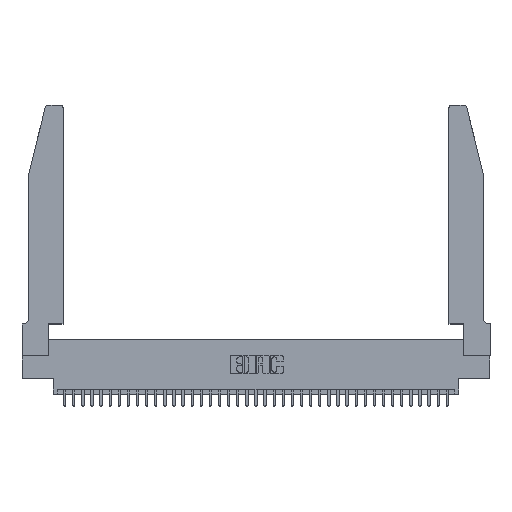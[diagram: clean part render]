
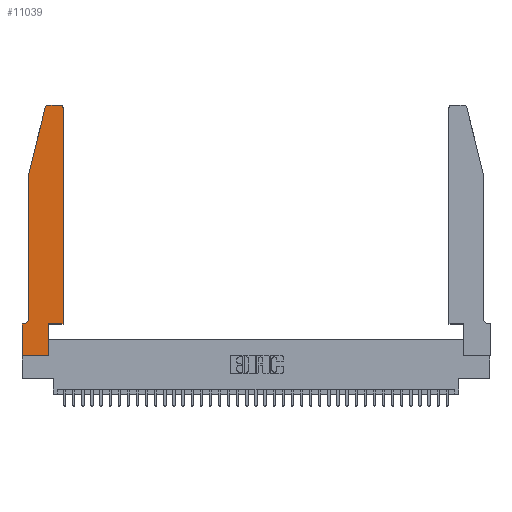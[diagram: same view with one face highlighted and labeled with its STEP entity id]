
A CAD part, top view. The second image highlights one B-rep face of the part: STEP entity #11039.
In plain terms, the highlighted planar face has unit normal (0, 0, 1).
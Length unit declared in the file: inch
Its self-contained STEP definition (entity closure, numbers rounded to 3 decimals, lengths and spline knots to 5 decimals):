
#48 = ORIENTED_EDGE ( 'NONE', *, *, #18609, .T. ) ;
#367 = ORIENTED_EDGE ( 'NONE', *, *, #29349, .T. ) ;
#1250 = CARTESIAN_POINT ( 'NONE',  ( 0.0755, 0.42, 0.37 ) ) ;
#1314 = VECTOR ( 'NONE', #4894, 39.37008 ) ;
#1820 = DIRECTION ( 'NONE',  ( -1., 0., 0. ) ) ;
#1969 = VERTEX_POINT ( 'NONE', #32398 ) ;
#2096 = LINE ( 'NONE', #29753, #17162 ) ;
#2302 = AXIS2_PLACEMENT_3D ( 'NONE', #9084, #29878, #12123 ) ;
#3725 = LINE ( 'NONE', #3844, #17818 ) ;
#3844 = CARTESIAN_POINT ( 'NONE',  ( 0., 0., 0.37 ) ) ;
#4588 = VECTOR ( 'NONE', #27755, 39.37008 ) ;
#4894 = DIRECTION ( 'NONE',  ( 0., 1., 0. ) ) ;
#4988 = VERTEX_POINT ( 'NONE', #13784 ) ;
#5032 = VERTEX_POINT ( 'NONE', #22776 ) ;
#5571 = CARTESIAN_POINT ( 'NONE',  ( 0.0755, 2., 0.37 ) ) ;
#5693 = CARTESIAN_POINT ( 'NONE',  ( 0., 0.35, 0.37 ) ) ;
#6256 = CARTESIAN_POINT ( 'NONE',  ( 0.4205, 2.72, 0.37 ) ) ;
#6925 = CARTESIAN_POINT ( 'NONE',  ( 0., 0., 0.37 ) ) ;
#7470 = EDGE_CURVE ( 'NONE', #35418, #28809, #28387, .T. ) ;
#8355 = ORIENTED_EDGE ( 'NONE', *, *, #7470, .T. ) ;
#8602 = LINE ( 'NONE', #31963, #14700 ) ;
#8677 = VECTOR ( 'NONE', #22527, 39.37008 ) ;
#8718 = DIRECTION ( 'NONE',  ( 0., 0., 1. ) ) ;
#9068 = AXIS2_PLACEMENT_3D ( 'NONE', #28570, #10781, #31528 ) ;
#9084 = CARTESIAN_POINT ( 'NONE',  ( 0.0055, 0.42, 0.37 ) ) ;
#9276 = DIRECTION ( 'NONE',  ( 1., 0., 0. ) ) ;
#9412 = CIRCLE ( 'NONE', #9068, 0.03 ) ;
#9448 = VERTEX_POINT ( 'NONE', #37239 ) ;
#10198 = EDGE_CURVE ( 'NONE', #10254, #31013, #8602, .T. ) ;
#10254 = VERTEX_POINT ( 'NONE', #5571 ) ;
#10673 = EDGE_CURVE ( 'NONE', #4988, #35418, #16707, .T. ) ;
#10781 = DIRECTION ( 'NONE',  ( 0., 0., 1. ) ) ;
#10873 = EDGE_CURVE ( 'NONE', #1969, #31015, #2096, .T. ) ;
#11039 = ADVANCED_FACE ( 'NONE', ( #13440 ), #23602, .T. ) ;
#11080 = CARTESIAN_POINT ( 'NONE',  ( 0.0755, 0.35, 0.37 ) ) ;
#12123 = DIRECTION ( 'NONE',  ( -1., 0., 0. ) ) ;
#13274 = CARTESIAN_POINT ( 'NONE',  ( 0.4505, 0.35, 0.37 ) ) ;
#13440 = FACE_OUTER_BOUND ( 'NONE', #13988, .T. ) ;
#13545 = CARTESIAN_POINT ( 'NONE',  ( 0.2605, 2.75, 0.37 ) ) ;
#13784 = CARTESIAN_POINT ( 'NONE',  ( 0.0055, 0.35, 0.37 ) ) ;
#13850 = CARTESIAN_POINT ( 'NONE',  ( 0.0755, 2., 0.37 ) ) ;
#13942 = ORIENTED_EDGE ( 'NONE', *, *, #18592, .T. ) ;
#13988 = EDGE_LOOP ( 'NONE', ( #367, #29294, #13942, #35464, #27269, #30937, #8355, #35736, #48, #34178, #27281, #27553 ) ) ;
#14250 = DIRECTION ( 'NONE',  ( 0., -1., 0. ) ) ;
#14700 = VECTOR ( 'NONE', #14250, 39.37008 ) ;
#14840 = EDGE_CURVE ( 'NONE', #9448, #34314, #9412, .T. ) ;
#16391 = LINE ( 'NONE', #28755, #1314 ) ;
#16707 = LINE ( 'NONE', #11080, #31525 ) ;
#16716 = EDGE_CURVE ( 'NONE', #31015, #5032, #37943, .T. ) ;
#17093 = EDGE_CURVE ( 'NONE', #31013, #4988, #34979, .T. ) ;
#17162 = VECTOR ( 'NONE', #32703, 39.37008 ) ;
#17196 = CARTESIAN_POINT ( 'NONE',  ( 0., 0., 0.37 ) ) ;
#17292 = CARTESIAN_POINT ( 'NONE',  ( 0.4505, 0.35, 0.37 ) ) ;
#17818 = VECTOR ( 'NONE', #24779, 39.37008 ) ;
#18349 = EDGE_CURVE ( 'NONE', #28809, #25086, #3725, .T. ) ;
#18592 = EDGE_CURVE ( 'NONE', #34314, #10254, #33052, .T. ) ;
#18609 = EDGE_CURVE ( 'NONE', #25086, #1969, #16391, .T. ) ;
#22527 = DIRECTION ( 'NONE',  ( -1., 0., 0. ) ) ;
#22776 = CARTESIAN_POINT ( 'NONE',  ( 0.4505, 2.72, 0.37 ) ) ;
#23157 = EDGE_CURVE ( 'NONE', #5032, #29342, #26316, .T. ) ;
#23602 = PLANE ( 'NONE',  #35067 ) ;
#24428 = CARTESIAN_POINT ( 'NONE',  ( 0.2865, 0., 0.37 ) ) ;
#24779 = DIRECTION ( 'NONE',  ( 1., 0., 0. ) ) ;
#25086 = VERTEX_POINT ( 'NONE', #24428 ) ;
#25229 = VECTOR ( 'NONE', #28625, 39.37008 ) ;
#26316 = CIRCLE ( 'NONE', #34104, 0.03 ) ;
#27121 = DIRECTION ( 'NONE',  ( 0., 0., 1. ) ) ;
#27269 = ORIENTED_EDGE ( 'NONE', *, *, #17093, .T. ) ;
#27281 = ORIENTED_EDGE ( 'NONE', *, *, #16716, .T. ) ;
#27553 = ORIENTED_EDGE ( 'NONE', *, *, #23157, .T. ) ;
#27755 = DIRECTION ( 'NONE',  ( 0., -1., 0. ) ) ;
#28387 = LINE ( 'NONE', #6925, #4588 ) ;
#28570 = CARTESIAN_POINT ( 'NONE',  ( 0.284, 2.72, 0.37 ) ) ;
#28625 = DIRECTION ( 'NONE',  ( -0.239, -0.971, 0. ) ) ;
#28701 = CARTESIAN_POINT ( 'NONE',  ( 0., 0.35, 0.37 ) ) ;
#28755 = CARTESIAN_POINT ( 'NONE',  ( 0.2865, 0.35, 0.37 ) ) ;
#28809 = VERTEX_POINT ( 'NONE', #17196 ) ;
#29294 = ORIENTED_EDGE ( 'NONE', *, *, #14840, .T. ) ;
#29342 = VERTEX_POINT ( 'NONE', #34196 ) ;
#29349 = EDGE_CURVE ( 'NONE', #29342, #9448, #33281, .T. ) ;
#29518 = DIRECTION ( 'NONE',  ( 1., 0., 0. ) ) ;
#29753 = CARTESIAN_POINT ( 'NONE',  ( 0.4505, 0.35, 0.37 ) ) ;
#29878 = DIRECTION ( 'NONE',  ( 0., 0., -1. ) ) ;
#30937 = ORIENTED_EDGE ( 'NONE', *, *, #10673, .T. ) ;
#31013 = VERTEX_POINT ( 'NONE', #1250 ) ;
#31015 = VERTEX_POINT ( 'NONE', #13274 ) ;
#31525 = VECTOR ( 'NONE', #1820, 39.37008 ) ;
#31528 = DIRECTION ( 'NONE',  ( 1., 0., 0. ) ) ;
#31963 = CARTESIAN_POINT ( 'NONE',  ( 0.0755, 2., 0.37 ) ) ;
#32009 = VECTOR ( 'NONE', #37899, 39.37008 ) ;
#32398 = CARTESIAN_POINT ( 'NONE',  ( 0.2865, 0.35, 0.37 ) ) ;
#32703 = DIRECTION ( 'NONE',  ( 1., 0., 0. ) ) ;
#33052 = LINE ( 'NONE', #13850, #25229 ) ;
#33281 = LINE ( 'NONE', #13545, #8677 ) ;
#34104 = AXIS2_PLACEMENT_3D ( 'NONE', #6256, #27121, #9276 ) ;
#34178 = ORIENTED_EDGE ( 'NONE', *, *, #10873, .T. ) ;
#34196 = CARTESIAN_POINT ( 'NONE',  ( 0.4205, 2.75, 0.37 ) ) ;
#34314 = VERTEX_POINT ( 'NONE', #37665 ) ;
#34979 = CIRCLE ( 'NONE', #2302, 0.07 ) ;
#35067 = AXIS2_PLACEMENT_3D ( 'NONE', #5693, #8718, #29518 ) ;
#35418 = VERTEX_POINT ( 'NONE', #28701 ) ;
#35464 = ORIENTED_EDGE ( 'NONE', *, *, #10198, .T. ) ;
#35736 = ORIENTED_EDGE ( 'NONE', *, *, #18349, .T. ) ;
#37239 = CARTESIAN_POINT ( 'NONE',  ( 0.284, 2.75, 0.37 ) ) ;
#37665 = CARTESIAN_POINT ( 'NONE',  ( 0.25487, 2.72718, 0.37 ) ) ;
#37899 = DIRECTION ( 'NONE',  ( 0., 1., 0. ) ) ;
#37943 = LINE ( 'NONE', #17292, #32009 ) ;
